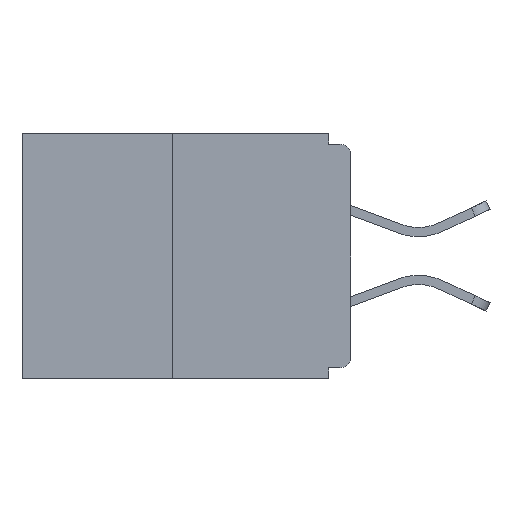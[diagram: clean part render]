
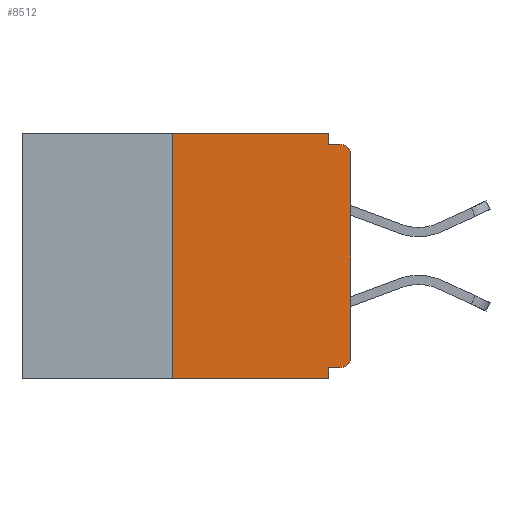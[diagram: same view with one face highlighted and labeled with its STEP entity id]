
A CAD part, left-side view. The second image highlights one B-rep face of the part: STEP entity #8512.
In plain terms, the highlighted planar face has unit normal (-1, 0, 0).
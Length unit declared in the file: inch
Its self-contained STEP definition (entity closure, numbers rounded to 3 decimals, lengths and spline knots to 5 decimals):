
#128 = ORIENTED_EDGE ( 'NONE', *, *, #14916, .F. ) ;
#150 = DIRECTION ( 'NONE',  ( 0., 1., 0. ) ) ;
#219 = LINE ( 'NONE', #2892, #720 ) ;
#368 = DIRECTION ( 'NONE',  ( 0., 0., -1. ) ) ;
#473 = DIRECTION ( 'NONE',  ( 1., 0., 0. ) ) ;
#575 = DIRECTION ( 'NONE',  ( 0., 0., -1. ) ) ;
#669 = EDGE_CURVE ( 'NONE', #12985, #5480, #17460, .T. ) ;
#720 = VECTOR ( 'NONE', #12354, 39.37008 ) ;
#997 = VERTEX_POINT ( 'NONE', #18418 ) ;
#1082 = CARTESIAN_POINT ( 'NONE',  ( 0., 0.015, -0.03 ) ) ;
#1305 = VECTOR ( 'NONE', #368, 39.37008 ) ;
#1306 = VERTEX_POINT ( 'NONE', #17169 ) ;
#1619 = CARTESIAN_POINT ( 'NONE',  ( 0., 0.25, -0.343 ) ) ;
#1775 = CARTESIAN_POINT ( 'NONE',  ( 0., 0.031, -0.343 ) ) ;
#1931 = DIRECTION ( 'NONE',  ( 0., 0., -1. ) ) ;
#2054 = CARTESIAN_POINT ( 'NONE',  ( 0., 0., -0.03 ) ) ;
#2188 = VERTEX_POINT ( 'NONE', #1619 ) ;
#2207 = VERTEX_POINT ( 'NONE', #18601 ) ;
#2251 = ORIENTED_EDGE ( 'NONE', *, *, #9888, .F. ) ;
#2892 = CARTESIAN_POINT ( 'NONE',  ( 0., 0., 0. ) ) ;
#3262 = CARTESIAN_POINT ( 'NONE',  ( 0., 0.25, 0. ) ) ;
#3402 = CARTESIAN_POINT ( 'NONE',  ( 0., 0., -0.015 ) ) ;
#4382 = EDGE_CURVE ( 'NONE', #5480, #15930, #219, .T. ) ;
#4452 = ORIENTED_EDGE ( 'NONE', *, *, #669, .T. ) ;
#4623 = FACE_OUTER_BOUND ( 'NONE', #9483, .T. ) ;
#4679 = ORIENTED_EDGE ( 'NONE', *, *, #4382, .T. ) ;
#5035 = DIRECTION ( 'NONE',  ( 0., -1., 0. ) ) ;
#5480 = VERTEX_POINT ( 'NONE', #9367 ) ;
#5530 = CARTESIAN_POINT ( 'NONE',  ( 0., 0.031, -0.328 ) ) ;
#6095 = CARTESIAN_POINT ( 'NONE',  ( 0., 0.015, -0.328 ) ) ;
#6373 = DIRECTION ( 'NONE',  ( 0., 0., 1. ) ) ;
#6706 = ORIENTED_EDGE ( 'NONE', *, *, #7200, .F. ) ;
#6912 = DIRECTION ( 'NONE',  ( 0., -1., 0. ) ) ;
#6977 = LINE ( 'NONE', #19044, #13024 ) ;
#7200 = EDGE_CURVE ( 'NONE', #11418, #2207, #12386, .T. ) ;
#7205 = DIRECTION ( 'NONE',  ( 0., 0., -1. ) ) ;
#8435 = EDGE_CURVE ( 'NONE', #1306, #997, #16434, .T. ) ;
#8512 = ADVANCED_FACE ( 'NONE', ( #4623 ), #9549, .F. ) ;
#9353 = AXIS2_PLACEMENT_3D ( 'NONE', #1082, #14762, #7205 ) ;
#9367 = CARTESIAN_POINT ( 'NONE',  ( 0., 0., -0.313 ) ) ;
#9374 = CARTESIAN_POINT ( 'NONE',  ( 0., 0., -0.328 ) ) ;
#9397 = DIRECTION ( 'NONE',  ( 0., 0., -1. ) ) ;
#9483 = EDGE_LOOP ( 'NONE', ( #128, #11354, #17607, #6706, #19988, #4452, #4679, #19097, #11230, #2251 ) ) ;
#9549 = PLANE ( 'NONE',  #15203 ) ;
#9840 = EDGE_CURVE ( 'NONE', #2188, #2207, #15644, .T. ) ;
#9888 = EDGE_CURVE ( 'NONE', #11872, #1306, #6977, .T. ) ;
#10367 = CARTESIAN_POINT ( 'NONE',  ( 0., 0.25, 0. ) ) ;
#10866 = CARTESIAN_POINT ( 'NONE',  ( 0., 0.031, 0. ) ) ;
#11121 = CARTESIAN_POINT ( 'NONE',  ( 0., 0.46, 0. ) ) ;
#11230 = ORIENTED_EDGE ( 'NONE', *, *, #8435, .F. ) ;
#11267 = CARTESIAN_POINT ( 'NONE',  ( 0., 0.46, 0. ) ) ;
#11354 = ORIENTED_EDGE ( 'NONE', *, *, #18372, .F. ) ;
#11418 = VERTEX_POINT ( 'NONE', #5530 ) ;
#11503 = AXIS2_PLACEMENT_3D ( 'NONE', #14133, #17077, #9397 ) ;
#11681 = EDGE_CURVE ( 'NONE', #15930, #997, #16813, .T. ) ;
#11841 = VECTOR ( 'NONE', #150, 39.37008 ) ;
#11872 = VERTEX_POINT ( 'NONE', #10866 ) ;
#12328 = VECTOR ( 'NONE', #5035, 39.37008 ) ;
#12354 = DIRECTION ( 'NONE',  ( 0., 0., 1. ) ) ;
#12386 = LINE ( 'NONE', #1775, #1305 ) ;
#12985 = VERTEX_POINT ( 'NONE', #6095 ) ;
#13024 = VECTOR ( 'NONE', #575, 39.37008 ) ;
#13433 = DIRECTION ( 'NONE',  ( 0., -1., 0. ) ) ;
#14133 = CARTESIAN_POINT ( 'NONE',  ( 0., 0.015, -0.313 ) ) ;
#14596 = VERTEX_POINT ( 'NONE', #10367 ) ;
#14754 = VECTOR ( 'NONE', #6373, 39.37008 ) ;
#14762 = DIRECTION ( 'NONE',  ( -1., 0., 0. ) ) ;
#14916 = EDGE_CURVE ( 'NONE', #14596, #11872, #19581, .T. ) ;
#14918 = VECTOR ( 'NONE', #6912, 39.37008 ) ;
#15203 = AXIS2_PLACEMENT_3D ( 'NONE', #11267, #473, #1931 ) ;
#15437 = EDGE_CURVE ( 'NONE', #12985, #11418, #16421, .T. ) ;
#15644 = LINE ( 'NONE', #17675, #14918 ) ;
#15930 = VERTEX_POINT ( 'NONE', #2054 ) ;
#15965 = VECTOR ( 'NONE', #13433, 39.37008 ) ;
#16421 = LINE ( 'NONE', #9374, #11841 ) ;
#16434 = LINE ( 'NONE', #3402, #12328 ) ;
#16813 = CIRCLE ( 'NONE', #9353, 0.015 ) ;
#17077 = DIRECTION ( 'NONE',  ( -1., 0., 0. ) ) ;
#17169 = CARTESIAN_POINT ( 'NONE',  ( 0., 0.031, -0.015 ) ) ;
#17460 = CIRCLE ( 'NONE', #11503, 0.015 ) ;
#17607 = ORIENTED_EDGE ( 'NONE', *, *, #9840, .T. ) ;
#17675 = CARTESIAN_POINT ( 'NONE',  ( 0., 0.46, -0.343 ) ) ;
#18372 = EDGE_CURVE ( 'NONE', #2188, #14596, #18855, .T. ) ;
#18418 = CARTESIAN_POINT ( 'NONE',  ( 0., 0.015, -0.015 ) ) ;
#18601 = CARTESIAN_POINT ( 'NONE',  ( 0., 0.031, -0.343 ) ) ;
#18855 = LINE ( 'NONE', #3262, #14754 ) ;
#19044 = CARTESIAN_POINT ( 'NONE',  ( 0., 0.031, 0. ) ) ;
#19097 = ORIENTED_EDGE ( 'NONE', *, *, #11681, .T. ) ;
#19581 = LINE ( 'NONE', #11121, #15965 ) ;
#19988 = ORIENTED_EDGE ( 'NONE', *, *, #15437, .F. ) ;
